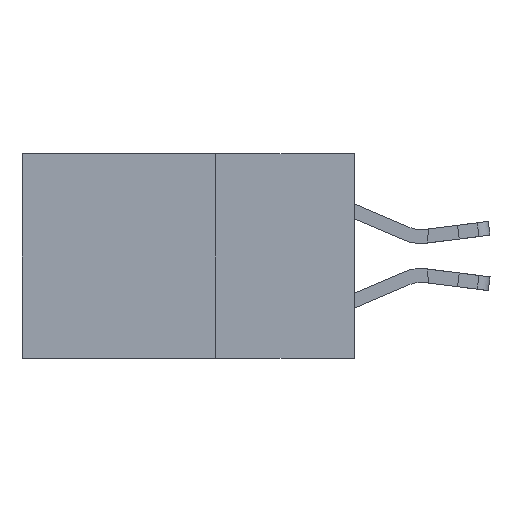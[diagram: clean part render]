
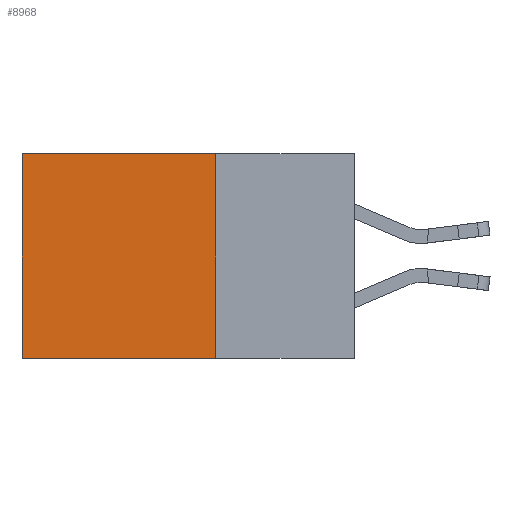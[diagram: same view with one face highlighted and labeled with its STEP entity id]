
A CAD part, left-side view. The second image highlights one B-rep face of the part: STEP entity #8968.
In plain terms, the highlighted planar face has unit normal (-1, 0, 0).
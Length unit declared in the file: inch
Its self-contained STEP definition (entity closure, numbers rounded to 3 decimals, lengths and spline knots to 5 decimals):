
#293 = ORIENTED_EDGE ( 'NONE', *, *, #17881, .F. ) ;
#1778 = DIRECTION ( 'NONE',  ( 0., 1., 0. ) ) ;
#2065 = PLANE ( 'NONE',  #11453 ) ;
#2174 = VECTOR ( 'NONE', #10074, 39.37008 ) ;
#2454 = EDGE_LOOP ( 'NONE', ( #14073, #293, #5706, #11338 ) ) ;
#2564 = DIRECTION ( 'NONE',  ( 0., 1., 0. ) ) ;
#3078 = VECTOR ( 'NONE', #1778, 39.37008 ) ;
#3862 = CARTESIAN_POINT ( 'NONE',  ( 0.2615, 0.6, -0.37 ) ) ;
#4088 = CARTESIAN_POINT ( 'NONE',  ( 0.2615, 0.25, 0. ) ) ;
#4521 = EDGE_CURVE ( 'NONE', #9939, #11274, #10005, .T. ) ;
#5029 = CARTESIAN_POINT ( 'NONE',  ( 0.2615, 0.25, -0.37 ) ) ;
#5706 = ORIENTED_EDGE ( 'NONE', *, *, #15834, .F. ) ;
#5776 = VECTOR ( 'NONE', #2564, 39.37008 ) ;
#6082 = LINE ( 'NONE', #18889, #2174 ) ;
#6515 = DIRECTION ( 'NONE',  ( 0., 0., -1. ) ) ;
#8423 = CARTESIAN_POINT ( 'NONE',  ( 0.2615, 0.25, -0.37 ) ) ;
#8968 = ADVANCED_FACE ( 'NONE', ( #16664 ), #2065, .F. ) ;
#9095 = EDGE_CURVE ( 'NONE', #11274, #11127, #11321, .T. ) ;
#9368 = CARTESIAN_POINT ( 'NONE',  ( 0.2615, 0.6, -0.37 ) ) ;
#9939 = VERTEX_POINT ( 'NONE', #4088 ) ;
#10005 = LINE ( 'NONE', #10581, #3078 ) ;
#10074 = DIRECTION ( 'NONE',  ( 0., 0., -1. ) ) ;
#10581 = CARTESIAN_POINT ( 'NONE',  ( 0.2615, 0.25, 0. ) ) ;
#11127 = VERTEX_POINT ( 'NONE', #9368 ) ;
#11274 = VERTEX_POINT ( 'NONE', #17063 ) ;
#11321 = LINE ( 'NONE', #3862, #14798 ) ;
#11326 = VERTEX_POINT ( 'NONE', #12804 ) ;
#11338 = ORIENTED_EDGE ( 'NONE', *, *, #4521, .T. ) ;
#11453 = AXIS2_PLACEMENT_3D ( 'NONE', #5029, #15355, #6515 ) ;
#12804 = CARTESIAN_POINT ( 'NONE',  ( 0.2615, 0.25, -0.37 ) ) ;
#14073 = ORIENTED_EDGE ( 'NONE', *, *, #9095, .T. ) ;
#14798 = VECTOR ( 'NONE', #15663, 39.37008 ) ;
#15355 = DIRECTION ( 'NONE',  ( 1., 0., 0. ) ) ;
#15663 = DIRECTION ( 'NONE',  ( 0., 0., -1. ) ) ;
#15834 = EDGE_CURVE ( 'NONE', #9939, #11326, #6082, .T. ) ;
#16664 = FACE_OUTER_BOUND ( 'NONE', #2454, .T. ) ;
#17063 = CARTESIAN_POINT ( 'NONE',  ( 0.2615, 0.6, 0. ) ) ;
#17088 = LINE ( 'NONE', #8423, #5776 ) ;
#17881 = EDGE_CURVE ( 'NONE', #11326, #11127, #17088, .T. ) ;
#18889 = CARTESIAN_POINT ( 'NONE',  ( 0.2615, 0.25, -0.37 ) ) ;
